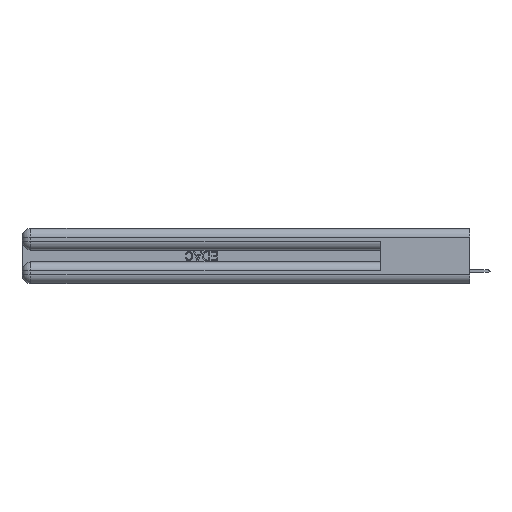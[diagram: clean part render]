
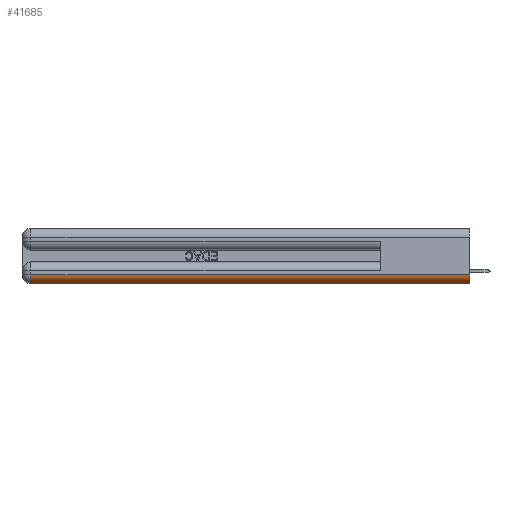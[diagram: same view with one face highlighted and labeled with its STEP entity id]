
A CAD part, left-side view. The second image highlights one B-rep face of the part: STEP entity #41685.
In plain terms, the highlighted cylindrical face has radius 1.524 mm (diameter 3.048 mm), a partial arc.
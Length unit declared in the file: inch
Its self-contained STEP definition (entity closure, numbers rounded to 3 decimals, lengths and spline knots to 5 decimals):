
#102 = LINE ( 'NONE', #40546, #19246 ) ;
#407 = DIRECTION ( 'NONE',  ( 0., -1., 0. ) ) ;
#936 = CARTESIAN_POINT ( 'NONE',  ( 0.06, 0., 0. ) ) ;
#2946 = CYLINDRICAL_SURFACE ( 'NONE', #10036, 0.06 ) ;
#7884 = CIRCLE ( 'NONE', #10001, 0.06 ) ;
#10001 = AXIS2_PLACEMENT_3D ( 'NONE', #21354, #18487, #27983 ) ;
#10036 = AXIS2_PLACEMENT_3D ( 'NONE', #26352, #16410, #25475 ) ;
#10346 = CARTESIAN_POINT ( 'NONE',  ( 0.06, 0., 0.06 ) ) ;
#11714 = CARTESIAN_POINT ( 'NONE',  ( 0., 2.94, 0.06 ) ) ;
#12844 = VERTEX_POINT ( 'NONE', #41108 ) ;
#14559 = ORIENTED_EDGE ( 'NONE', *, *, #22727, .F. ) ;
#16410 = DIRECTION ( 'NONE',  ( 0., 1., 0. ) ) ;
#17260 = EDGE_LOOP ( 'NONE', ( #40859, #36466, #19285, #14559 ) ) ;
#18487 = DIRECTION ( 'NONE',  ( 0., 1., 0. ) ) ;
#18835 = CARTESIAN_POINT ( 'NONE',  ( 0., 0., 0.06 ) ) ;
#19246 = VECTOR ( 'NONE', #29928, 39.37008 ) ;
#19285 = ORIENTED_EDGE ( 'NONE', *, *, #41050, .F. ) ;
#19726 = FACE_OUTER_BOUND ( 'NONE', #17260, .T. ) ;
#20258 = VERTEX_POINT ( 'NONE', #936 ) ;
#21354 = CARTESIAN_POINT ( 'NONE',  ( 0.06, 2.94, 0.06 ) ) ;
#22727 = EDGE_CURVE ( 'NONE', #20258, #12844, #42356, .T. ) ;
#23629 = VERTEX_POINT ( 'NONE', #18835 ) ;
#23941 = VERTEX_POINT ( 'NONE', #11714 ) ;
#25475 = DIRECTION ( 'NONE',  ( 0., 0., 1. ) ) ;
#25621 = CIRCLE ( 'NONE', #41148, 0.06 ) ;
#26352 = CARTESIAN_POINT ( 'NONE',  ( 0.06, 0., 0.06 ) ) ;
#27338 = DIRECTION ( 'NONE',  ( 0., 0., 1. ) ) ;
#27983 = DIRECTION ( 'NONE',  ( 0., 0., 1. ) ) ;
#28650 = CARTESIAN_POINT ( 'NONE',  ( 0.06, 3., 0. ) ) ;
#29928 = DIRECTION ( 'NONE',  ( 0., -1., 0. ) ) ;
#31191 = VECTOR ( 'NONE', #35283, 39.37008 ) ;
#35078 = EDGE_CURVE ( 'NONE', #23629, #20258, #25621, .T. ) ;
#35283 = DIRECTION ( 'NONE',  ( 0., 1., 0. ) ) ;
#36466 = ORIENTED_EDGE ( 'NONE', *, *, #43575, .F. ) ;
#40546 = CARTESIAN_POINT ( 'NONE',  ( 0., 0., 0.06 ) ) ;
#40859 = ORIENTED_EDGE ( 'NONE', *, *, #35078, .F. ) ;
#41050 = EDGE_CURVE ( 'NONE', #12844, #23941, #7884, .T. ) ;
#41108 = CARTESIAN_POINT ( 'NONE',  ( 0.06, 2.94, 0. ) ) ;
#41148 = AXIS2_PLACEMENT_3D ( 'NONE', #10346, #407, #27338 ) ;
#41685 = ADVANCED_FACE ( 'NONE', ( #19726 ), #2946, .T. ) ;
#42356 = LINE ( 'NONE', #28650, #31191 ) ;
#43575 = EDGE_CURVE ( 'NONE', #23941, #23629, #102, .T. ) ;
